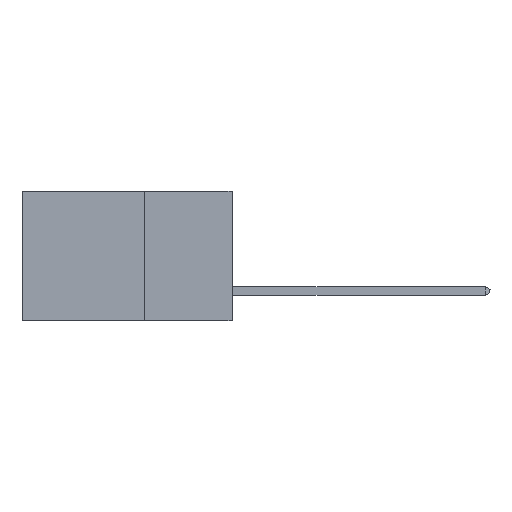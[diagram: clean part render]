
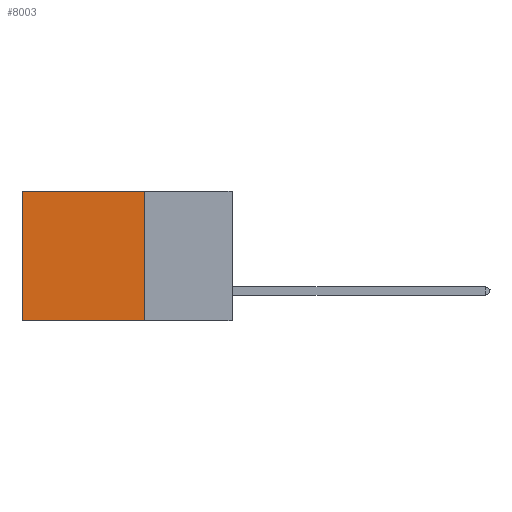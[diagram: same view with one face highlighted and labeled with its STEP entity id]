
A CAD part, left-side view. The second image highlights one B-rep face of the part: STEP entity #8003.
In plain terms, the highlighted planar face has unit normal (-1, 0, 0).
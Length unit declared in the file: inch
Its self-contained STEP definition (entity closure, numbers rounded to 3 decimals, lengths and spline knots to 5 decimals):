
#465 = VECTOR ( 'NONE', #14145, 39.37008 ) ;
#736 = DIRECTION ( 'NONE',  ( 1., 0., 0. ) ) ;
#1379 = VERTEX_POINT ( 'NONE', #3048 ) ;
#1423 = CARTESIAN_POINT ( 'NONE',  ( 0.2875, 0.25, -0.37 ) ) ;
#1831 = CARTESIAN_POINT ( 'NONE',  ( 0.2875, 0.25, 0. ) ) ;
#2083 = EDGE_LOOP ( 'NONE', ( #6922, #16244, #11678, #4798 ) ) ;
#2347 = LINE ( 'NONE', #1831, #465 ) ;
#2374 = DIRECTION ( 'NONE',  ( 0., 1., 0. ) ) ;
#3048 = CARTESIAN_POINT ( 'NONE',  ( 0.2875, 0.25, 0. ) ) ;
#3187 = EDGE_CURVE ( 'NONE', #14559, #6357, #10558, .T. ) ;
#3848 = EDGE_CURVE ( 'NONE', #1379, #14559, #2347, .T. ) ;
#3989 = EDGE_CURVE ( 'NONE', #1379, #14898, #14572, .T. ) ;
#4380 = VECTOR ( 'NONE', #2374, 39.37008 ) ;
#4589 = LINE ( 'NONE', #13136, #4380 ) ;
#4798 = ORIENTED_EDGE ( 'NONE', *, *, #3848, .T. ) ;
#5214 = DIRECTION ( 'NONE',  ( 0., 0., -1. ) ) ;
#5501 = FACE_OUTER_BOUND ( 'NONE', #2083, .T. ) ;
#6357 = VERTEX_POINT ( 'NONE', #13221 ) ;
#6922 = ORIENTED_EDGE ( 'NONE', *, *, #3187, .T. ) ;
#6978 = VECTOR ( 'NONE', #11194, 39.37008 ) ;
#7025 = PLANE ( 'NONE',  #9989 ) ;
#8003 = ADVANCED_FACE ( 'NONE', ( #5501 ), #7025, .F. ) ;
#9989 = AXIS2_PLACEMENT_3D ( 'NONE', #16464, #736, #12877 ) ;
#10425 = EDGE_CURVE ( 'NONE', #14898, #6357, #4589, .T. ) ;
#10558 = LINE ( 'NONE', #14112, #6978 ) ;
#10564 = CARTESIAN_POINT ( 'NONE',  ( 0.2875, 0.25, 0. ) ) ;
#11194 = DIRECTION ( 'NONE',  ( 0., 0., -1. ) ) ;
#11678 = ORIENTED_EDGE ( 'NONE', *, *, #3989, .F. ) ;
#12877 = DIRECTION ( 'NONE',  ( 0., 0., -1. ) ) ;
#13136 = CARTESIAN_POINT ( 'NONE',  ( 0.2875, 0.25, -0.37 ) ) ;
#13221 = CARTESIAN_POINT ( 'NONE',  ( 0.2875, 0.6, -0.37 ) ) ;
#14112 = CARTESIAN_POINT ( 'NONE',  ( 0.2875, 0.6, 0. ) ) ;
#14145 = DIRECTION ( 'NONE',  ( 0., 1., 0. ) ) ;
#14559 = VERTEX_POINT ( 'NONE', #17101 ) ;
#14572 = LINE ( 'NONE', #10564, #17095 ) ;
#14898 = VERTEX_POINT ( 'NONE', #1423 ) ;
#16244 = ORIENTED_EDGE ( 'NONE', *, *, #10425, .F. ) ;
#16464 = CARTESIAN_POINT ( 'NONE',  ( 0.2875, 0.25, 0. ) ) ;
#17095 = VECTOR ( 'NONE', #5214, 39.37008 ) ;
#17101 = CARTESIAN_POINT ( 'NONE',  ( 0.2875, 0.6, 0. ) ) ;
